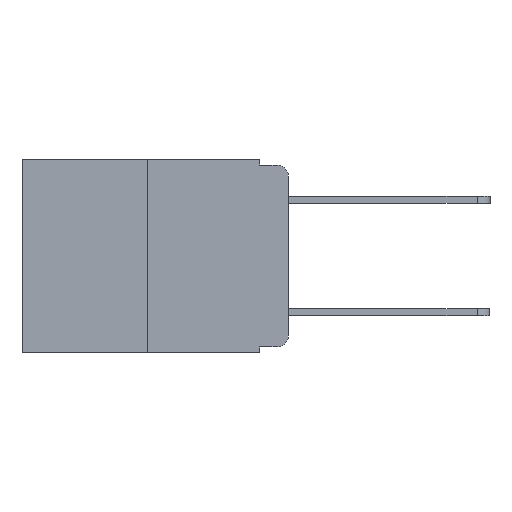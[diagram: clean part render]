
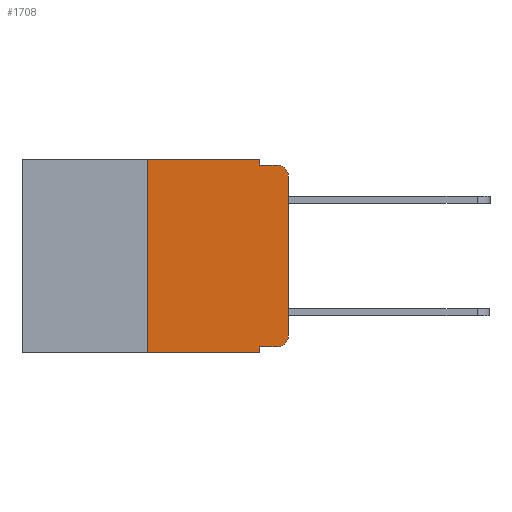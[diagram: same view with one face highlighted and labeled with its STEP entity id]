
A CAD part, left-side view. The second image highlights one B-rep face of the part: STEP entity #1708.
In plain terms, the highlighted planar face has unit normal (-1, 0, 0).
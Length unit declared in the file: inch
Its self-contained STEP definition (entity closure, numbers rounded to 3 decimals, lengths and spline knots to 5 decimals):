
#159 = CARTESIAN_POINT ( 'NONE',  ( 0., 0.051, -0.333 ) ) ;
#289 = VERTEX_POINT ( 'NONE', #5084 ) ;
#622 = ORIENTED_EDGE ( 'NONE', *, *, #8835, .T. ) ;
#697 = ORIENTED_EDGE ( 'NONE', *, *, #8838, .T. ) ;
#1636 = ORIENTED_EDGE ( 'NONE', *, *, #8841, .F. ) ;
#1708 = ADVANCED_FACE ( 'NONE', ( #16508 ), #13709, .F. ) ;
#1741 = ORIENTED_EDGE ( 'NONE', *, *, #8857, .F. ) ;
#1932 = ORIENTED_EDGE ( 'NONE', *, *, #8132, .F. ) ;
#1979 = ORIENTED_EDGE ( 'NONE', *, *, #8862, .F. ) ;
#1983 = DIRECTION ( 'NONE',  ( -1., 0., 0. ) ) ;
#2055 = DIRECTION ( 'NONE',  ( 0., 0., -1. ) ) ;
#2121 = VERTEX_POINT ( 'NONE', #6570 ) ;
#2125 = DIRECTION ( 'NONE',  ( -1., 0., 0. ) ) ;
#2151 = ORIENTED_EDGE ( 'NONE', *, *, #8451, .T. ) ;
#2367 = CARTESIAN_POINT ( 'NONE',  ( 0., 0.051, -0.01 ) ) ;
#2424 = VERTEX_POINT ( 'NONE', #3192 ) ;
#2660 = ORIENTED_EDGE ( 'NONE', *, *, #8870, .F. ) ;
#2843 = ORIENTED_EDGE ( 'NONE', *, *, #8888, .T. ) ;
#2994 = VECTOR ( 'NONE', #16097, 39.37008 ) ;
#3015 = ORIENTED_EDGE ( 'NONE', *, *, #8891, .T. ) ;
#3192 = CARTESIAN_POINT ( 'NONE',  ( 0., 0.02, -0.01 ) ) ;
#3282 = VECTOR ( 'NONE', #8808, 39.37008 ) ;
#3723 = CARTESIAN_POINT ( 'NONE',  ( 0., 0., 0. ) ) ;
#3845 = LINE ( 'NONE', #7166, #3282 ) ;
#5084 = CARTESIAN_POINT ( 'NONE',  ( 0., 0.051, -0.333 ) ) ;
#5453 = CARTESIAN_POINT ( 'NONE',  ( 0., 0.051, -0.01 ) ) ;
#6570 = CARTESIAN_POINT ( 'NONE',  ( 0., 0., -0.313 ) ) ;
#7166 = CARTESIAN_POINT ( 'NONE',  ( 0., 0.051, 0. ) ) ;
#7227 = DIRECTION ( 'NONE',  ( 0., -1., 0. ) ) ;
#7243 = CIRCLE ( 'NONE', #16962, 0.02 ) ;
#7391 = CARTESIAN_POINT ( 'NONE',  ( 0., 0.051, -0.343 ) ) ;
#7712 = LINE ( 'NONE', #18542, #11498 ) ;
#7738 = CARTESIAN_POINT ( 'NONE',  ( 0., 0.051, 0. ) ) ;
#8132 = EDGE_CURVE ( 'NONE', #12887, #11349, #11719, .T. ) ;
#8248 = LINE ( 'NONE', #5453, #18988 ) ;
#8309 = DIRECTION ( 'NONE',  ( 0., -1., 0. ) ) ;
#8451 = EDGE_CURVE ( 'NONE', #14604, #15411, #16346, .T. ) ;
#8808 = DIRECTION ( 'NONE',  ( 0., 0., -1. ) ) ;
#8835 = EDGE_CURVE ( 'NONE', #2121, #16308, #19404, .T. ) ;
#8838 = EDGE_CURVE ( 'NONE', #16308, #2424, #15919, .T. ) ;
#8841 = EDGE_CURVE ( 'NONE', #16573, #2424, #8248, .T. ) ;
#8857 = EDGE_CURVE ( 'NONE', #11349, #16573, #3845, .T. ) ;
#8862 = EDGE_CURVE ( 'NONE', #14604, #12887, #7712, .T. ) ;
#8870 = EDGE_CURVE ( 'NONE', #289, #15411, #15500, .T. ) ;
#8888 = EDGE_CURVE ( 'NONE', #289, #17085, #18174, .T. ) ;
#8891 = EDGE_CURVE ( 'NONE', #17085, #2121, #7243, .T. ) ;
#10434 = CARTESIAN_POINT ( 'NONE',  ( 0., 0.051, 0. ) ) ;
#11173 = CARTESIAN_POINT ( 'NONE',  ( 0., 0.25, 0. ) ) ;
#11349 = VERTEX_POINT ( 'NONE', #7738 ) ;
#11498 = VECTOR ( 'NONE', #11894, 39.37008 ) ;
#11719 = LINE ( 'NONE', #14750, #2994 ) ;
#11839 = CARTESIAN_POINT ( 'NONE',  ( 0., 0.02, -0.03 ) ) ;
#11894 = DIRECTION ( 'NONE',  ( 0., 0., 1. ) ) ;
#11955 = CARTESIAN_POINT ( 'NONE',  ( 0., 0.02, -0.313 ) ) ;
#12305 = VECTOR ( 'NONE', #15853, 39.37008 ) ;
#12887 = VERTEX_POINT ( 'NONE', #11173 ) ;
#12968 = CARTESIAN_POINT ( 'NONE',  ( 0., 0.473, 0. ) ) ;
#13167 = DIRECTION ( 'NONE',  ( 0., 0., -1. ) ) ;
#13265 = DIRECTION ( 'NONE',  ( 0., 0., -1. ) ) ;
#13709 = PLANE ( 'NONE',  #19115 ) ;
#14018 = DIRECTION ( 'NONE',  ( 1., 0., 0. ) ) ;
#14327 = CARTESIAN_POINT ( 'NONE',  ( 0., 0., -0.03 ) ) ;
#14439 = CARTESIAN_POINT ( 'NONE',  ( 0., 0.02, -0.333 ) ) ;
#14497 = DIRECTION ( 'NONE',  ( 0., -1., 0. ) ) ;
#14604 = VERTEX_POINT ( 'NONE', #15472 ) ;
#14648 = VECTOR ( 'NONE', #7227, 39.37008 ) ;
#14724 = DIRECTION ( 'NONE',  ( 0., 0., -1. ) ) ;
#14750 = CARTESIAN_POINT ( 'NONE',  ( 0., 0.473, 0. ) ) ;
#15070 = VECTOR ( 'NONE', #2055, 39.37008 ) ;
#15411 = VERTEX_POINT ( 'NONE', #7391 ) ;
#15472 = CARTESIAN_POINT ( 'NONE',  ( 0., 0.25, -0.343 ) ) ;
#15500 = LINE ( 'NONE', #10434, #15070 ) ;
#15853 = DIRECTION ( 'NONE',  ( 0., 0., 1. ) ) ;
#15919 = CIRCLE ( 'NONE', #16067, 0.02 ) ;
#16067 = AXIS2_PLACEMENT_3D ( 'NONE', #11839, #1983, #13167 ) ;
#16097 = DIRECTION ( 'NONE',  ( 0., -1., 0. ) ) ;
#16308 = VERTEX_POINT ( 'NONE', #14327 ) ;
#16346 = LINE ( 'NONE', #16908, #19426 ) ;
#16444 = EDGE_LOOP ( 'NONE', ( #622, #697, #1636, #1741, #1932, #1979, #2151, #2660, #2843, #3015 ) ) ;
#16508 = FACE_OUTER_BOUND ( 'NONE', #16444, .T. ) ;
#16573 = VERTEX_POINT ( 'NONE', #2367 ) ;
#16908 = CARTESIAN_POINT ( 'NONE',  ( 0., 0.473, -0.343 ) ) ;
#16962 = AXIS2_PLACEMENT_3D ( 'NONE', #11955, #2125, #13265 ) ;
#17085 = VERTEX_POINT ( 'NONE', #14439 ) ;
#18174 = LINE ( 'NONE', #159, #14648 ) ;
#18542 = CARTESIAN_POINT ( 'NONE',  ( 0., 0.25, 0. ) ) ;
#18988 = VECTOR ( 'NONE', #14497, 39.37008 ) ;
#19115 = AXIS2_PLACEMENT_3D ( 'NONE', #12968, #14018, #14724 ) ;
#19404 = LINE ( 'NONE', #3723, #12305 ) ;
#19426 = VECTOR ( 'NONE', #8309, 39.37008 ) ;
